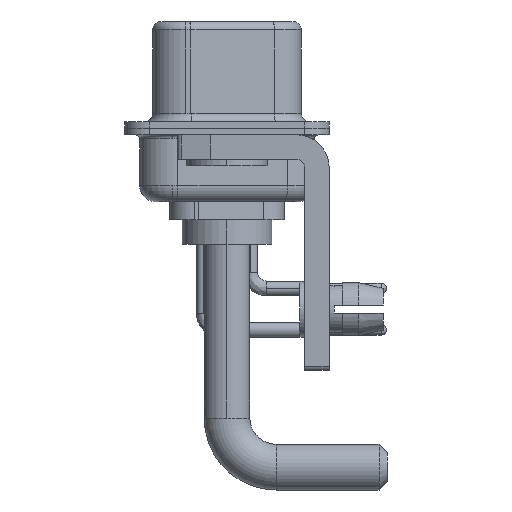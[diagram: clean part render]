
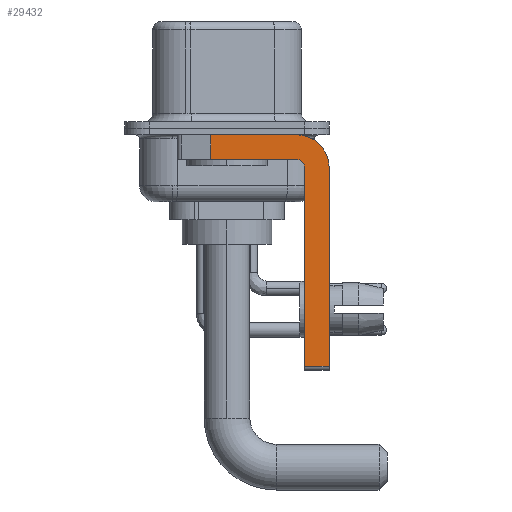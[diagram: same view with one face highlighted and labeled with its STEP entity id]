
A CAD part, left-side view. The second image highlights one B-rep face of the part: STEP entity #29432.
In plain terms, the highlighted planar face has unit normal (-1, 0, 0).
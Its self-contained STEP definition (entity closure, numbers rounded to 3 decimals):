
#463 = CARTESIAN_POINT ( 'NONE',  ( -2.9, -4.25, -2.4 ) ) ;
#505 = LINE ( 'NONE', #10008, #2567 ) ;
#1167 = VECTOR ( 'NONE', #20383, 1000. ) ;
#1868 = ORIENTED_EDGE ( 'NONE', *, *, #11527, .F. ) ;
#2189 = CARTESIAN_POINT ( 'NONE',  ( -2.9, -4.25, -1.9 ) ) ;
#2502 = ORIENTED_EDGE ( 'NONE', *, *, #11799, .T. ) ;
#2567 = VECTOR ( 'NONE', #29119, 1000. ) ;
#3268 = CARTESIAN_POINT ( 'NONE',  ( -2.9, -6.25, -2.4 ) ) ;
#3270 = VECTOR ( 'NONE', #17706, 1000. ) ;
#4527 = CARTESIAN_POINT ( 'NONE',  ( -2.9, -4.75, -14.55 ) ) ;
#4578 = CARTESIAN_POINT ( 'NONE',  ( -2.9, -4.25, -2.4 ) ) ;
#5025 = CIRCLE ( 'NONE', #13005, 0.5 ) ;
#5683 = VERTEX_POINT ( 'NONE', #24919 ) ;
#6478 = ORIENTED_EDGE ( 'NONE', *, *, #21122, .F. ) ;
#6605 = DIRECTION ( 'NONE',  ( 1., 0., 0. ) ) ;
#6653 = CIRCLE ( 'NONE', #9096, 2. ) ;
#7090 = ORIENTED_EDGE ( 'NONE', *, *, #14929, .F. ) ;
#7349 = CARTESIAN_POINT ( 'NONE',  ( -2.9, 0.978, -0.4 ) ) ;
#7552 = EDGE_LOOP ( 'NONE', ( #25891, #2502, #22410, #1868, #18738, #25342, #7090, #6478 ) ) ;
#7971 = LINE ( 'NONE', #17866, #3270 ) ;
#8030 = VERTEX_POINT ( 'NONE', #30212 ) ;
#8558 = LINE ( 'NONE', #3268, #28701 ) ;
#8794 = CARTESIAN_POINT ( 'NONE',  ( -2.9, 3., -0.4 ) ) ;
#8860 = VERTEX_POINT ( 'NONE', #19368 ) ;
#8944 = EDGE_CURVE ( 'NONE', #10420, #29378, #16026, .T. ) ;
#9096 = AXIS2_PLACEMENT_3D ( 'NONE', #4578, #6605, #21193 ) ;
#9605 = VECTOR ( 'NONE', #18379, 1000. ) ;
#10008 = CARTESIAN_POINT ( 'NONE',  ( -2.9, 0.978, -1.9 ) ) ;
#10420 = VERTEX_POINT ( 'NONE', #7349 ) ;
#10936 = VERTEX_POINT ( 'NONE', #29490 ) ;
#11123 = VERTEX_POINT ( 'NONE', #26203 ) ;
#11527 = EDGE_CURVE ( 'NONE', #8860, #11123, #5025, .T. ) ;
#11799 = EDGE_CURVE ( 'NONE', #10420, #8030, #505, .T. ) ;
#11827 = EDGE_CURVE ( 'NONE', #18383, #8860, #13140, .T. ) ;
#12816 = DIRECTION ( 'NONE',  ( 0., 0., -1. ) ) ;
#13005 = AXIS2_PLACEMENT_3D ( 'NONE', #25700, #28351, #30395 ) ;
#13140 = LINE ( 'NONE', #20031, #30555 ) ;
#13940 = EDGE_CURVE ( 'NONE', #11123, #8030, #16429, .T. ) ;
#13956 = AXIS2_PLACEMENT_3D ( 'NONE', #463, #29073, #19989 ) ;
#14929 = EDGE_CURVE ( 'NONE', #10936, #5683, #8558, .T. ) ;
#16026 = LINE ( 'NONE', #8794, #9605 ) ;
#16429 = LINE ( 'NONE', #2189, #1167 ) ;
#17042 = FACE_OUTER_BOUND ( 'NONE', #7552, .T. ) ;
#17534 = DIRECTION ( 'NONE',  ( 0., 0., 1. ) ) ;
#17706 = DIRECTION ( 'NONE',  ( 0., -1., 0. ) ) ;
#17866 = CARTESIAN_POINT ( 'NONE',  ( -2.9, -4.25, -14.55 ) ) ;
#18379 = DIRECTION ( 'NONE',  ( 0., -1., 0. ) ) ;
#18383 = VERTEX_POINT ( 'NONE', #4527 ) ;
#18738 = ORIENTED_EDGE ( 'NONE', *, *, #11827, .F. ) ;
#19368 = CARTESIAN_POINT ( 'NONE',  ( -2.9, -4.75, -2.4 ) ) ;
#19989 = DIRECTION ( 'NONE',  ( 0., 0., -1. ) ) ;
#20031 = CARTESIAN_POINT ( 'NONE',  ( -2.9, -4.75, -14.8 ) ) ;
#20383 = DIRECTION ( 'NONE',  ( 0., 1., 0. ) ) ;
#21122 = EDGE_CURVE ( 'NONE', #29378, #10936, #6653, .T. ) ;
#21193 = DIRECTION ( 'NONE',  ( 0., 0., -1. ) ) ;
#22338 = PLANE ( 'NONE',  #13956 ) ;
#22410 = ORIENTED_EDGE ( 'NONE', *, *, #13940, .F. ) ;
#24825 = CARTESIAN_POINT ( 'NONE',  ( -2.9, -4.25, -0.4 ) ) ;
#24859 = EDGE_CURVE ( 'NONE', #18383, #5683, #7971, .T. ) ;
#24919 = CARTESIAN_POINT ( 'NONE',  ( -2.9, -6.25, -14.55 ) ) ;
#25342 = ORIENTED_EDGE ( 'NONE', *, *, #24859, .T. ) ;
#25700 = CARTESIAN_POINT ( 'NONE',  ( -2.9, -4.25, -2.4 ) ) ;
#25891 = ORIENTED_EDGE ( 'NONE', *, *, #8944, .F. ) ;
#26203 = CARTESIAN_POINT ( 'NONE',  ( -2.9, -4.25, -1.9 ) ) ;
#28351 = DIRECTION ( 'NONE',  ( -1., 0., 0. ) ) ;
#28701 = VECTOR ( 'NONE', #12816, 1000. ) ;
#29073 = DIRECTION ( 'NONE',  ( 1., 0., 0. ) ) ;
#29119 = DIRECTION ( 'NONE',  ( 0., 0., -1. ) ) ;
#29378 = VERTEX_POINT ( 'NONE', #24825 ) ;
#29432 = ADVANCED_FACE ( 'NONE', ( #17042 ), #22338, .F. ) ;
#29490 = CARTESIAN_POINT ( 'NONE',  ( -2.9, -6.25, -2.4 ) ) ;
#30212 = CARTESIAN_POINT ( 'NONE',  ( -2.9, 0.978, -1.9 ) ) ;
#30395 = DIRECTION ( 'NONE',  ( 0., 0., 1. ) ) ;
#30555 = VECTOR ( 'NONE', #17534, 1000. ) ;
